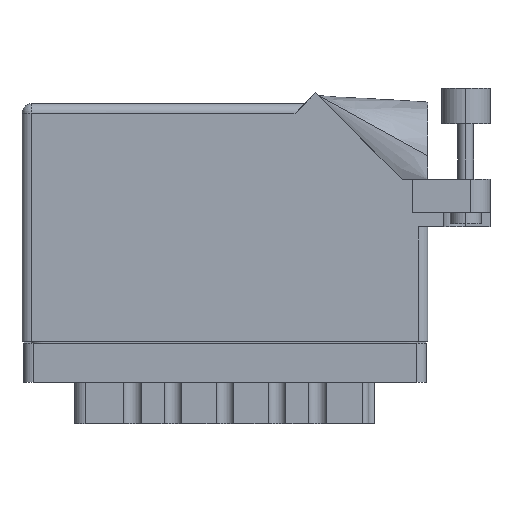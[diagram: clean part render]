
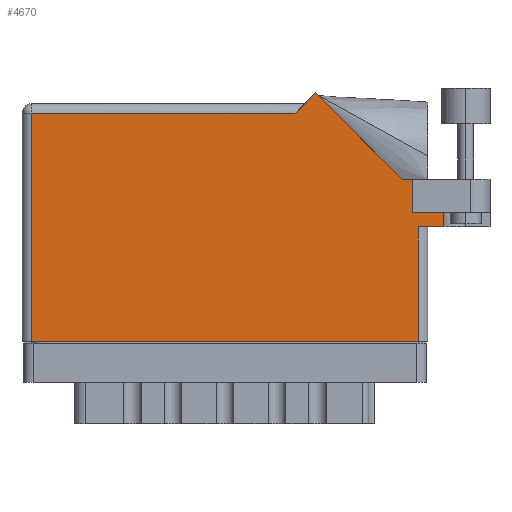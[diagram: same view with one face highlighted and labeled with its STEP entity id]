
A CAD part, front view. The second image highlights one B-rep face of the part: STEP entity #4670.
In plain terms, the highlighted face is planar.
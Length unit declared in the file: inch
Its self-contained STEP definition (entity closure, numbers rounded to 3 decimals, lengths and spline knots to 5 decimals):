
#284 = CARTESIAN_POINT ( 'NONE',  ( 3.012, 1.044, 0. ) ) ;
#1396 = DIRECTION ( 'NONE',  ( -1., 0., 0. ) ) ;
#1563 = CARTESIAN_POINT ( 'NONE',  ( 0., 1.53, 0. ) ) ;
#2091 = VERTEX_POINT ( 'NONE', #47865 ) ;
#2198 = CARTESIAN_POINT ( 'NONE',  ( 0., 1.468, 0. ) ) ;
#2584 = LINE ( 'NONE', #31800, #23167 ) ;
#2796 = EDGE_CURVE ( 'NONE', #28579, #2091, #33893, .T. ) ;
#3109 = LINE ( 'NONE', #46341, #27250 ) ;
#3191 = ORIENTED_EDGE ( 'NONE', *, *, #48576, .T. ) ;
#4082 = FACE_OUTER_BOUND ( 'NONE', #19347, .T. ) ;
#4127 = CARTESIAN_POINT ( 'NONE',  ( 1.757, 1.468, 0. ) ) ;
#4670 = ADVANCED_FACE ( 'NONE', ( #4082 ), #43636, .F. ) ;
#5150 = EDGE_CURVE ( 'NONE', #17141, #27756, #11708, .T. ) ;
#5331 = VECTOR ( 'NONE', #16098, 39.37008 ) ;
#6508 = EDGE_CURVE ( 'NONE', #43364, #20459, #32711, .T. ) ;
#6608 = LINE ( 'NONE', #19362, #43386 ) ;
#7305 = ORIENTED_EDGE ( 'NONE', *, *, #45464, .T. ) ;
#7967 = CARTESIAN_POINT ( 'NONE',  ( 1.819, 1.53, 0. ) ) ;
#8019 = LINE ( 'NONE', #36541, #41213 ) ;
#8336 = VERTEX_POINT ( 'NONE', #34079 ) ;
#8573 = CARTESIAN_POINT ( 'NONE',  ( 2.7135, 0.831, 0. ) ) ;
#10138 = ORIENTED_EDGE ( 'NONE', *, *, #6508, .F. ) ;
#10320 = ORIENTED_EDGE ( 'NONE', *, *, #39469, .T. ) ;
#10338 = LINE ( 'NONE', #10644, #39294 ) ;
#10644 = CARTESIAN_POINT ( 'NONE',  ( 2.512, 0.831, 0. ) ) ;
#11708 = LINE ( 'NONE', #284, #26229 ) ;
#11724 = ORIENTED_EDGE ( 'NONE', *, *, #12991, .T. ) ;
#12991 = EDGE_CURVE ( 'NONE', #2091, #8336, #3109, .T. ) ;
#15160 = DIRECTION ( 'NONE',  ( -1., 0., 0. ) ) ;
#15628 = LINE ( 'NONE', #7967, #5331 ) ;
#16098 = DIRECTION ( 'NONE',  ( -0.707, -0.707, 0. ) ) ;
#16220 = AXIS2_PLACEMENT_3D ( 'NONE', #1563, #43462, #1396 ) ;
#16554 = EDGE_CURVE ( 'NONE', #27523, #17141, #10338, .T. ) ;
#17141 = VERTEX_POINT ( 'NONE', #45669 ) ;
#17836 = ORIENTED_EDGE ( 'NONE', *, *, #33272, .T. ) ;
#18452 = CARTESIAN_POINT ( 'NONE',  ( 2.44642, 1.044, 0. ) ) ;
#18793 = DIRECTION ( 'NONE',  ( -0.707, 0.707, 0. ) ) ;
#19347 = EDGE_LOOP ( 'NONE', ( #7305, #10320, #3191, #10138, #32807, #47109, #34410, #23237, #17836, #39093, #11724 ) ) ;
#19362 = CARTESIAN_POINT ( 'NONE',  ( 0., 0., 0. ) ) ;
#20459 = VERTEX_POINT ( 'NONE', #31504 ) ;
#22563 = CARTESIAN_POINT ( 'NONE',  ( 2.512, 0.831, 0. ) ) ;
#23167 = VECTOR ( 'NONE', #31633, 39.37008 ) ;
#23237 = ORIENTED_EDGE ( 'NONE', *, *, #49394, .T. ) ;
#23687 = VECTOR ( 'NONE', #32965, 39.37008 ) ;
#23903 = VECTOR ( 'NONE', #29957, 39.37008 ) ;
#24618 = CARTESIAN_POINT ( 'NONE',  ( 1.88971, 1.60071, 0. ) ) ;
#26085 = VECTOR ( 'NONE', #15160, 39.37008 ) ;
#26229 = VECTOR ( 'NONE', #38665, 39.37008 ) ;
#27250 = VECTOR ( 'NONE', #34862, 39.37008 ) ;
#27523 = VERTEX_POINT ( 'NONE', #33753 ) ;
#27756 = VERTEX_POINT ( 'NONE', #44009 ) ;
#28579 = VERTEX_POINT ( 'NONE', #4127 ) ;
#28722 = LINE ( 'NONE', #22563, #23903 ) ;
#29957 = DIRECTION ( 'NONE',  ( 1., 0., 0. ) ) ;
#31504 = CARTESIAN_POINT ( 'NONE',  ( 2.7135, 0.737, 0. ) ) ;
#31633 = DIRECTION ( 'NONE',  ( 0., 1., 0. ) ) ;
#31737 = VERTEX_POINT ( 'NONE', #37246 ) ;
#31800 = CARTESIAN_POINT ( 'NONE',  ( 2.55, 0.737, 0. ) ) ;
#32711 = LINE ( 'NONE', #48092, #23687 ) ;
#32807 = ORIENTED_EDGE ( 'NONE', *, *, #42469, .F. ) ;
#32965 = DIRECTION ( 'NONE',  ( 0., -1., 0. ) ) ;
#33272 = EDGE_CURVE ( 'NONE', #48435, #28579, #15628, .T. ) ;
#33352 = LINE ( 'NONE', #18452, #36909 ) ;
#33753 = CARTESIAN_POINT ( 'NONE',  ( 2.512, 0.831, 0. ) ) ;
#33893 = LINE ( 'NONE', #2198, #26085 ) ;
#34079 = CARTESIAN_POINT ( 'NONE',  ( 0.062, 0., 0. ) ) ;
#34410 = ORIENTED_EDGE ( 'NONE', *, *, #5150, .T. ) ;
#34862 = DIRECTION ( 'NONE',  ( 0., -1., 0. ) ) ;
#36541 = CARTESIAN_POINT ( 'NONE',  ( 2.612, 0.737, 0. ) ) ;
#36909 = VECTOR ( 'NONE', #18793, 39.37008 ) ;
#37246 = CARTESIAN_POINT ( 'NONE',  ( 2.55, 0.737, 0. ) ) ;
#37427 = CARTESIAN_POINT ( 'NONE',  ( 2.55, 0., 0. ) ) ;
#38665 = DIRECTION ( 'NONE',  ( -1., 0., 0. ) ) ;
#39093 = ORIENTED_EDGE ( 'NONE', *, *, #2796, .T. ) ;
#39294 = VECTOR ( 'NONE', #41297, 39.37008 ) ;
#39469 = EDGE_CURVE ( 'NONE', #44574, #31737, #2584, .T. ) ;
#41213 = VECTOR ( 'NONE', #48805, 39.37008 ) ;
#41297 = DIRECTION ( 'NONE',  ( 0., 1., 0. ) ) ;
#42469 = EDGE_CURVE ( 'NONE', #27523, #43364, #28722, .T. ) ;
#42745 = DIRECTION ( 'NONE',  ( 1., 0., 0. ) ) ;
#43364 = VERTEX_POINT ( 'NONE', #8573 ) ;
#43386 = VECTOR ( 'NONE', #42745, 39.37008 ) ;
#43462 = DIRECTION ( 'NONE',  ( 0., 0., -1. ) ) ;
#43636 = PLANE ( 'NONE',  #16220 ) ;
#44009 = CARTESIAN_POINT ( 'NONE',  ( 2.44642, 1.044, 0. ) ) ;
#44574 = VERTEX_POINT ( 'NONE', #37427 ) ;
#45464 = EDGE_CURVE ( 'NONE', #8336, #44574, #6608, .T. ) ;
#45669 = CARTESIAN_POINT ( 'NONE',  ( 2.512, 1.044, 0. ) ) ;
#46341 = CARTESIAN_POINT ( 'NONE',  ( 0.062, 0., 0. ) ) ;
#47109 = ORIENTED_EDGE ( 'NONE', *, *, #16554, .T. ) ;
#47865 = CARTESIAN_POINT ( 'NONE',  ( 0.062, 1.468, 0. ) ) ;
#48092 = CARTESIAN_POINT ( 'NONE',  ( 2.7135, 1.16177, 0. ) ) ;
#48435 = VERTEX_POINT ( 'NONE', #24618 ) ;
#48576 = EDGE_CURVE ( 'NONE', #31737, #20459, #8019, .T. ) ;
#48805 = DIRECTION ( 'NONE',  ( 1., 0., 0. ) ) ;
#49394 = EDGE_CURVE ( 'NONE', #27756, #48435, #33352, .T. ) ;
